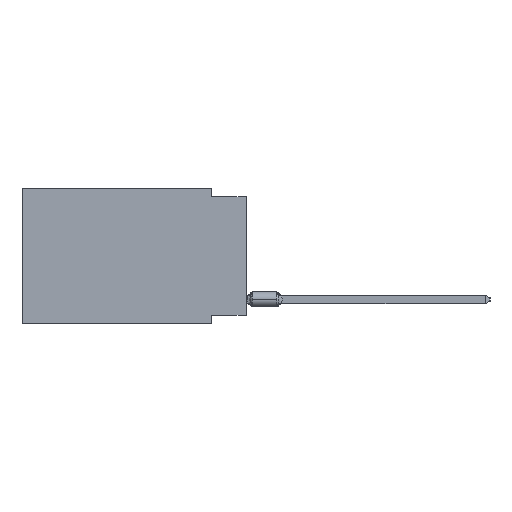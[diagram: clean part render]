
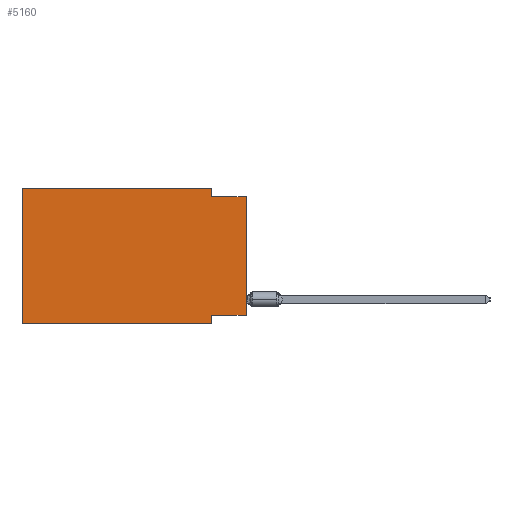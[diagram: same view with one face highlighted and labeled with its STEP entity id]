
A CAD part, left-side view. The second image highlights one B-rep face of the part: STEP entity #5160.
In plain terms, the highlighted planar face has unit normal (-1, 0, 0).
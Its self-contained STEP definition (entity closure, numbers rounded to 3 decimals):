
#886 = VECTOR ( 'NONE', #49924, 1000. ) ;
#1085 = DIRECTION ( 'NONE',  ( 0., 0., -1. ) ) ;
#1427 = VECTOR ( 'NONE', #3852, 1000. ) ;
#1606 = ORIENTED_EDGE ( 'NONE', *, *, #40243, .T. ) ;
#3106 = LINE ( 'NONE', #26674, #886 ) ;
#3852 = DIRECTION ( 'NONE',  ( 0., 0., 1. ) ) ;
#4672 = CARTESIAN_POINT ( 'NONE',  ( 0., 0., -0.635 ) ) ;
#5160 = ADVANCED_FACE ( 'NONE', ( #40620 ), #5419, .F. ) ;
#5419 = PLANE ( 'NONE',  #8198 ) ;
#5858 = VECTOR ( 'NONE', #15469, 1000. ) ;
#6687 = EDGE_CURVE ( 'NONE', #24986, #29307, #44176, .T. ) ;
#8198 = AXIS2_PLACEMENT_3D ( 'NONE', #21465, #9308, #37256 ) ;
#8927 = CARTESIAN_POINT ( 'NONE',  ( 0., 16.383, 0. ) ) ;
#9230 = LINE ( 'NONE', #33285, #34884 ) ;
#9308 = DIRECTION ( 'NONE',  ( 1., 0., 0. ) ) ;
#9492 = CARTESIAN_POINT ( 'NONE',  ( 0., 0., -9.271 ) ) ;
#9901 = VECTOR ( 'NONE', #45860, 1000. ) ;
#12068 = EDGE_CURVE ( 'NONE', #37923, #45766, #9230, .T. ) ;
#15469 = DIRECTION ( 'NONE',  ( 0., 0., 1. ) ) ;
#15546 = ORIENTED_EDGE ( 'NONE', *, *, #19468, .F. ) ;
#15662 = EDGE_CURVE ( 'NONE', #34507, #18690, #50812, .T. ) ;
#16388 = VERTEX_POINT ( 'NONE', #44281 ) ;
#18690 = VERTEX_POINT ( 'NONE', #46933 ) ;
#18707 = DIRECTION ( 'NONE',  ( 0., 0., -1. ) ) ;
#19468 = EDGE_CURVE ( 'NONE', #18690, #29307, #3106, .T. ) ;
#19818 = DIRECTION ( 'NONE',  ( 0., -1., 0. ) ) ;
#19896 = CARTESIAN_POINT ( 'NONE',  ( 0., 16.383, 0. ) ) ;
#21465 = CARTESIAN_POINT ( 'NONE',  ( 0., 16.383, 0. ) ) ;
#22619 = EDGE_CURVE ( 'NONE', #16388, #34507, #27829, .T. ) ;
#22622 = ORIENTED_EDGE ( 'NONE', *, *, #12068, .F. ) ;
#23843 = ORIENTED_EDGE ( 'NONE', *, *, #49335, .F. ) ;
#24124 = CARTESIAN_POINT ( 'NONE',  ( 0., 2.54, 0. ) ) ;
#24772 = LINE ( 'NONE', #9492, #32258 ) ;
#24810 = CARTESIAN_POINT ( 'NONE',  ( 0., 16.383, -9.906 ) ) ;
#24986 = VERTEX_POINT ( 'NONE', #34161 ) ;
#25280 = ORIENTED_EDGE ( 'NONE', *, *, #22619, .F. ) ;
#26674 = CARTESIAN_POINT ( 'NONE',  ( 0., 0., -0.635 ) ) ;
#26744 = CARTESIAN_POINT ( 'NONE',  ( 0., 16.383, -9.906 ) ) ;
#26920 = VECTOR ( 'NONE', #1085, 1000. ) ;
#27829 = LINE ( 'NONE', #8927, #32984 ) ;
#29057 = CARTESIAN_POINT ( 'NONE',  ( 0., 2.54, 0. ) ) ;
#29307 = VERTEX_POINT ( 'NONE', #4672 ) ;
#29643 = VERTEX_POINT ( 'NONE', #24810 ) ;
#32258 = VECTOR ( 'NONE', #48272, 1000. ) ;
#32984 = VECTOR ( 'NONE', #19818, 1000. ) ;
#33285 = CARTESIAN_POINT ( 'NONE',  ( 0., 2.54, -9.906 ) ) ;
#34161 = CARTESIAN_POINT ( 'NONE',  ( 0., 0., -9.271 ) ) ;
#34507 = VERTEX_POINT ( 'NONE', #29057 ) ;
#34816 = CARTESIAN_POINT ( 'NONE',  ( 0., 2.54, -9.906 ) ) ;
#34884 = VECTOR ( 'NONE', #18707, 1000. ) ;
#35680 = LINE ( 'NONE', #19896, #1427 ) ;
#37256 = DIRECTION ( 'NONE',  ( 0., 0., -1. ) ) ;
#37923 = VERTEX_POINT ( 'NONE', #38937 ) ;
#38937 = CARTESIAN_POINT ( 'NONE',  ( 0., 2.54, -9.271 ) ) ;
#40243 = EDGE_CURVE ( 'NONE', #29643, #45766, #45615, .T. ) ;
#40620 = FACE_OUTER_BOUND ( 'NONE', #45958, .T. ) ;
#40939 = EDGE_CURVE ( 'NONE', #24986, #37923, #24772, .T. ) ;
#43875 = ORIENTED_EDGE ( 'NONE', *, *, #40939, .F. ) ;
#44045 = ORIENTED_EDGE ( 'NONE', *, *, #15662, .F. ) ;
#44176 = LINE ( 'NONE', #50881, #5858 ) ;
#44281 = CARTESIAN_POINT ( 'NONE',  ( 0., 16.383, 0. ) ) ;
#45360 = ORIENTED_EDGE ( 'NONE', *, *, #6687, .T. ) ;
#45615 = LINE ( 'NONE', #26744, #9901 ) ;
#45766 = VERTEX_POINT ( 'NONE', #34816 ) ;
#45860 = DIRECTION ( 'NONE',  ( 0., -1., 0. ) ) ;
#45958 = EDGE_LOOP ( 'NONE', ( #45360, #15546, #44045, #25280, #23843, #1606, #22622, #43875 ) ) ;
#46933 = CARTESIAN_POINT ( 'NONE',  ( 0., 2.54, -0.635 ) ) ;
#48272 = DIRECTION ( 'NONE',  ( 0., 1., 0. ) ) ;
#49335 = EDGE_CURVE ( 'NONE', #29643, #16388, #35680, .T. ) ;
#49924 = DIRECTION ( 'NONE',  ( 0., -1., 0. ) ) ;
#50812 = LINE ( 'NONE', #24124, #26920 ) ;
#50881 = CARTESIAN_POINT ( 'NONE',  ( 0., 0., 0. ) ) ;
